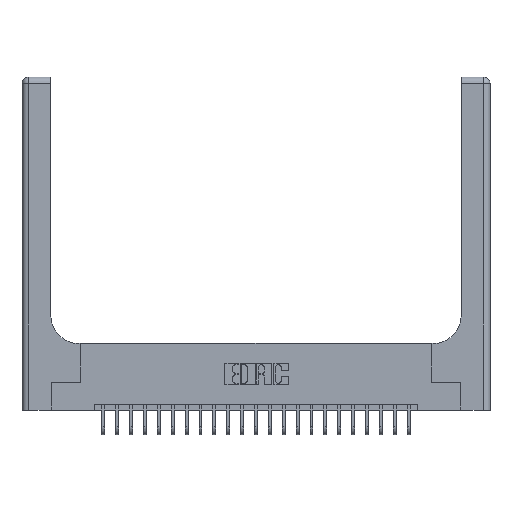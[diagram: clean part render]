
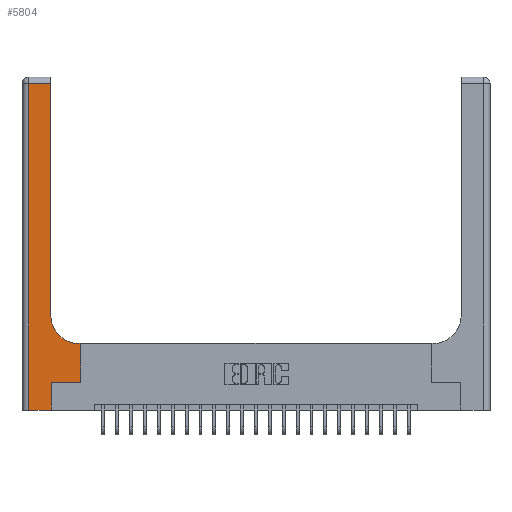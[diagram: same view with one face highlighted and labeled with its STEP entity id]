
A CAD part, top view. The second image highlights one B-rep face of the part: STEP entity #5804.
In plain terms, the highlighted planar face has unit normal (0, 0, 1).
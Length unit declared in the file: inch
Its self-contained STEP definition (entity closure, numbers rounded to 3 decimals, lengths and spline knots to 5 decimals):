
#160 = ORIENTED_EDGE ( 'NONE', *, *, #13831, .T. ) ;
#170 = VERTEX_POINT ( 'NONE', #2958 ) ;
#460 = DIRECTION ( 'NONE',  ( -1., 0., 0. ) ) ;
#466 = ORIENTED_EDGE ( 'NONE', *, *, #17845, .T. ) ;
#1145 = EDGE_CURVE ( 'NONE', #4343, #5261, #2150, .T. ) ;
#1324 = ORIENTED_EDGE ( 'NONE', *, *, #11370, .T. ) ;
#1374 = LINE ( 'NONE', #21045, #21835 ) ;
#1547 = DIRECTION ( 'NONE',  ( 0., 1., 0. ) ) ;
#1548 = DIRECTION ( 'NONE',  ( 0., 1., 0. ) ) ;
#1651 = VECTOR ( 'NONE', #1548, 39.37008 ) ;
#1685 = VECTOR ( 'NONE', #23588, 39.37008 ) ;
#1767 = LINE ( 'NONE', #18730, #5896 ) ;
#1840 = EDGE_CURVE ( 'NONE', #7601, #21231, #14587, .T. ) ;
#1851 = CARTESIAN_POINT ( 'NONE',  ( 0.528, 0.6, 0.37 ) ) ;
#2112 = CARTESIAN_POINT ( 'NONE',  ( 0.265, 0.25, 0.37 ) ) ;
#2150 = LINE ( 'NONE', #2274, #11381 ) ;
#2274 = CARTESIAN_POINT ( 'NONE',  ( 0.26, 0.6, 0.37 ) ) ;
#2958 = CARTESIAN_POINT ( 'NONE',  ( 0.26, 2.94, 0.37 ) ) ;
#3047 = AXIS2_PLACEMENT_3D ( 'NONE', #8134, #15790, #8320 ) ;
#3753 = CARTESIAN_POINT ( 'NONE',  ( 0.528, 0.25, 0.37 ) ) ;
#4197 = CARTESIAN_POINT ( 'NONE',  ( 0.06, 0., 0.37 ) ) ;
#4343 = VERTEX_POINT ( 'NONE', #1851 ) ;
#4461 = CARTESIAN_POINT ( 'NONE',  ( 0.26, 3., 0.37 ) ) ;
#4678 = EDGE_CURVE ( 'NONE', #24501, #15325, #1374, .T. ) ;
#5261 = VERTEX_POINT ( 'NONE', #5575 ) ;
#5575 = CARTESIAN_POINT ( 'NONE',  ( 0.51, 0.6, 0.37 ) ) ;
#5804 = ADVANCED_FACE ( 'NONE', ( #15273 ), #8088, .F. ) ;
#5863 = ORIENTED_EDGE ( 'NONE', *, *, #1840, .T. ) ;
#5896 = VECTOR ( 'NONE', #10952, 39.37008 ) ;
#6191 = VERTEX_POINT ( 'NONE', #3753 ) ;
#6269 = LINE ( 'NONE', #8016, #12817 ) ;
#7601 = VERTEX_POINT ( 'NONE', #24350 ) ;
#8007 = ORIENTED_EDGE ( 'NONE', *, *, #11937, .T. ) ;
#8016 = CARTESIAN_POINT ( 'NONE',  ( 0., 2.94, 0.37 ) ) ;
#8088 = PLANE ( 'NONE',  #10298 ) ;
#8134 = CARTESIAN_POINT ( 'NONE',  ( 0.51, 0.85, 0.37 ) ) ;
#8240 = CIRCLE ( 'NONE', #3047, 0.25 ) ;
#8320 = DIRECTION ( 'NONE',  ( 1., 0., 0. ) ) ;
#8590 = DIRECTION ( 'NONE',  ( 0., -1., 0. ) ) ;
#9021 = ORIENTED_EDGE ( 'NONE', *, *, #1145, .T. ) ;
#9380 = LINE ( 'NONE', #4461, #1685 ) ;
#9809 = CARTESIAN_POINT ( 'NONE',  ( 0.06, 2.94, 0.37 ) ) ;
#10298 = AXIS2_PLACEMENT_3D ( 'NONE', #23510, #19727, #23674 ) ;
#10430 = ORIENTED_EDGE ( 'NONE', *, *, #20392, .T. ) ;
#10952 = DIRECTION ( 'NONE',  ( 1., 0., 0. ) ) ;
#11370 = EDGE_CURVE ( 'NONE', #21866, #170, #9380, .T. ) ;
#11381 = VECTOR ( 'NONE', #460, 39.37008 ) ;
#11658 = VECTOR ( 'NONE', #1547, 39.37008 ) ;
#11937 = EDGE_CURVE ( 'NONE', #15325, #7601, #22714, .T. ) ;
#12618 = LINE ( 'NONE', #12902, #1651 ) ;
#12817 = VECTOR ( 'NONE', #13696, 39.37008 ) ;
#12902 = CARTESIAN_POINT ( 'NONE',  ( 0.528, 0.25, 0.37 ) ) ;
#13152 = CARTESIAN_POINT ( 'NONE',  ( 0.26, 0.85, 0.37 ) ) ;
#13458 = EDGE_LOOP ( 'NONE', ( #1324, #466, #13786, #8007, #5863, #10430, #22180, #9021, #160 ) ) ;
#13538 = VECTOR ( 'NONE', #16620, 39.37008 ) ;
#13696 = DIRECTION ( 'NONE',  ( -1., 0., 0. ) ) ;
#13786 = ORIENTED_EDGE ( 'NONE', *, *, #4678, .T. ) ;
#13831 = EDGE_CURVE ( 'NONE', #5261, #21866, #8240, .T. ) ;
#14587 = LINE ( 'NONE', #21946, #11658 ) ;
#15273 = FACE_OUTER_BOUND ( 'NONE', #13458, .T. ) ;
#15325 = VERTEX_POINT ( 'NONE', #4197 ) ;
#15790 = DIRECTION ( 'NONE',  ( 0., 0., -1. ) ) ;
#16620 = DIRECTION ( 'NONE',  ( 1., 0., 0. ) ) ;
#17845 = EDGE_CURVE ( 'NONE', #170, #24501, #6269, .T. ) ;
#18730 = CARTESIAN_POINT ( 'NONE',  ( 0.265, 0.25, 0.37 ) ) ;
#19727 = DIRECTION ( 'NONE',  ( 0., 0., -1. ) ) ;
#20392 = EDGE_CURVE ( 'NONE', #21231, #6191, #1767, .T. ) ;
#21045 = CARTESIAN_POINT ( 'NONE',  ( 0.06, 3., 0.37 ) ) ;
#21231 = VERTEX_POINT ( 'NONE', #2112 ) ;
#21835 = VECTOR ( 'NONE', #8590, 39.37008 ) ;
#21866 = VERTEX_POINT ( 'NONE', #13152 ) ;
#21946 = CARTESIAN_POINT ( 'NONE',  ( 0.265, 0., 0.37 ) ) ;
#22180 = ORIENTED_EDGE ( 'NONE', *, *, #23734, .T. ) ;
#22264 = CARTESIAN_POINT ( 'NONE',  ( 0., 0., 0.37 ) ) ;
#22714 = LINE ( 'NONE', #22264, #13538 ) ;
#23510 = CARTESIAN_POINT ( 'NONE',  ( 0., 3., 0.37 ) ) ;
#23588 = DIRECTION ( 'NONE',  ( 0., 1., 0. ) ) ;
#23674 = DIRECTION ( 'NONE',  ( -1., 0., 0. ) ) ;
#23734 = EDGE_CURVE ( 'NONE', #6191, #4343, #12618, .T. ) ;
#24350 = CARTESIAN_POINT ( 'NONE',  ( 0.265, 0., 0.37 ) ) ;
#24501 = VERTEX_POINT ( 'NONE', #9809 ) ;
